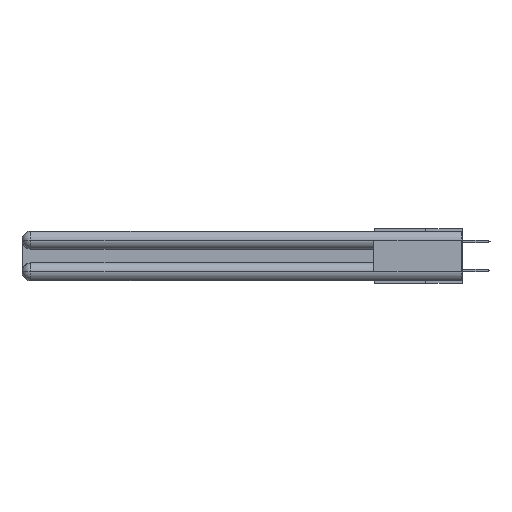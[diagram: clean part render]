
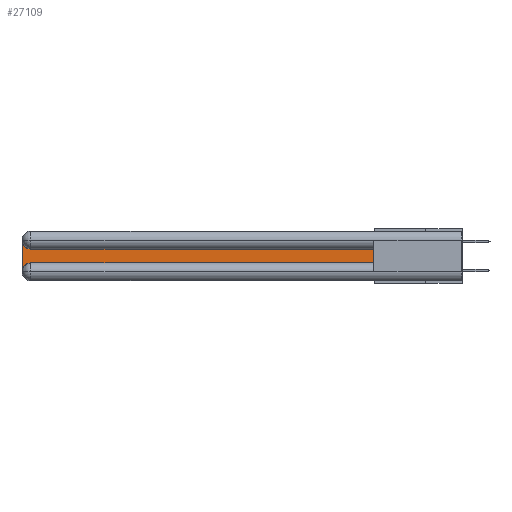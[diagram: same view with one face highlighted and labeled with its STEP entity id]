
A CAD part, left-side view. The second image highlights one B-rep face of the part: STEP entity #27109.
In plain terms, the highlighted planar face has unit normal (-1, 0, 0).
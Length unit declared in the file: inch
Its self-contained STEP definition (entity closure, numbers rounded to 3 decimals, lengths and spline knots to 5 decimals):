
#145 = ORIENTED_EDGE ( 'NONE', *, *, #27965, .T. ) ;
#1100 = DIRECTION ( 'NONE',  ( 0., -1., 0. ) ) ;
#2671 = AXIS2_PLACEMENT_3D ( 'NONE', #33255, #27286, #10962 ) ;
#2889 = ORIENTED_EDGE ( 'NONE', *, *, #33209, .T. ) ;
#3701 = CARTESIAN_POINT ( 'NONE',  ( 0.075, 3., -0.0625 ) ) ;
#3821 = VERTEX_POINT ( 'NONE', #16174 ) ;
#5636 = VECTOR ( 'NONE', #18697, 39.37008 ) ;
#7103 = CARTESIAN_POINT ( 'NONE',  ( 0.075, 0.6, -0.2175 ) ) ;
#8862 = EDGE_CURVE ( 'NONE', #11841, #17387, #18624, .T. ) ;
#9509 = AXIS2_PLACEMENT_3D ( 'NONE', #29408, #32179, #34917 ) ;
#10359 = ORIENTED_EDGE ( 'NONE', *, *, #24891, .T. ) ;
#10962 = DIRECTION ( 'NONE',  ( 0., 0., -1. ) ) ;
#11056 = CARTESIAN_POINT ( 'NONE',  ( 0.075, 2.94, -0.1225 ) ) ;
#11841 = VERTEX_POINT ( 'NONE', #17378 ) ;
#12059 = CARTESIAN_POINT ( 'NONE',  ( 0.075, 0.6, -0.2175 ) ) ;
#12852 = CARTESIAN_POINT ( 'NONE',  ( 0.075, 0.6, -0.1225 ) ) ;
#12912 = DIRECTION ( 'NONE',  ( 1., 0., 0. ) ) ;
#13939 = VECTOR ( 'NONE', #15083, 39.37008 ) ;
#14587 = CIRCLE ( 'NONE', #9509, 0.06 ) ;
#15083 = DIRECTION ( 'NONE',  ( 0., 0., 1. ) ) ;
#15916 = PLANE ( 'NONE',  #28633 ) ;
#16174 = CARTESIAN_POINT ( 'NONE',  ( 0.075, 0.6, -0.1225 ) ) ;
#16362 = FACE_OUTER_BOUND ( 'NONE', #26389, .T. ) ;
#16526 = LINE ( 'NONE', #23099, #13939 ) ;
#17378 = CARTESIAN_POINT ( 'NONE',  ( 0.075, 2.94, -0.2175 ) ) ;
#17387 = VERTEX_POINT ( 'NONE', #7103 ) ;
#18267 = VECTOR ( 'NONE', #26559, 39.37008 ) ;
#18624 = LINE ( 'NONE', #12059, #27529 ) ;
#18697 = DIRECTION ( 'NONE',  ( 0., 0., -1. ) ) ;
#18700 = DIRECTION ( 'NONE',  ( 0., 0., -1. ) ) ;
#18793 = ORIENTED_EDGE ( 'NONE', *, *, #30242, .T. ) ;
#20218 = LINE ( 'NONE', #34985, #5636 ) ;
#20270 = ORIENTED_EDGE ( 'NONE', *, *, #8862, .T. ) ;
#22453 = CIRCLE ( 'NONE', #2671, 0.06 ) ;
#23099 = CARTESIAN_POINT ( 'NONE',  ( 0.075, 0.6, -0.2175 ) ) ;
#24799 = VERTEX_POINT ( 'NONE', #3701 ) ;
#24891 = EDGE_CURVE ( 'NONE', #3821, #32409, #31019, .T. ) ;
#26389 = EDGE_LOOP ( 'NONE', ( #10359, #145, #31529, #18793, #20270, #2889 ) ) ;
#26545 = CARTESIAN_POINT ( 'NONE',  ( 0.075, 3., -0.2775 ) ) ;
#26559 = DIRECTION ( 'NONE',  ( 0., 1., 0. ) ) ;
#26977 = CARTESIAN_POINT ( 'NONE',  ( 0.075, 3., -0.1225 ) ) ;
#27109 = ADVANCED_FACE ( 'NONE', ( #16362 ), #15916, .F. ) ;
#27286 = DIRECTION ( 'NONE',  ( 1., 0., 0. ) ) ;
#27529 = VECTOR ( 'NONE', #1100, 39.37008 ) ;
#27965 = EDGE_CURVE ( 'NONE', #32409, #24799, #22453, .T. ) ;
#28284 = VERTEX_POINT ( 'NONE', #26545 ) ;
#28633 = AXIS2_PLACEMENT_3D ( 'NONE', #26977, #12912, #18700 ) ;
#29137 = EDGE_CURVE ( 'NONE', #24799, #28284, #20218, .T. ) ;
#29408 = CARTESIAN_POINT ( 'NONE',  ( 0.075, 2.94, -0.2775 ) ) ;
#30242 = EDGE_CURVE ( 'NONE', #28284, #11841, #14587, .T. ) ;
#31019 = LINE ( 'NONE', #12852, #18267 ) ;
#31529 = ORIENTED_EDGE ( 'NONE', *, *, #29137, .T. ) ;
#32179 = DIRECTION ( 'NONE',  ( 1., 0., 0. ) ) ;
#32409 = VERTEX_POINT ( 'NONE', #11056 ) ;
#33209 = EDGE_CURVE ( 'NONE', #17387, #3821, #16526, .T. ) ;
#33255 = CARTESIAN_POINT ( 'NONE',  ( 0.075, 2.94, -0.0625 ) ) ;
#34917 = DIRECTION ( 'NONE',  ( 0., 0., -1. ) ) ;
#34985 = CARTESIAN_POINT ( 'NONE',  ( 0.075, 3., -0.2175 ) ) ;
